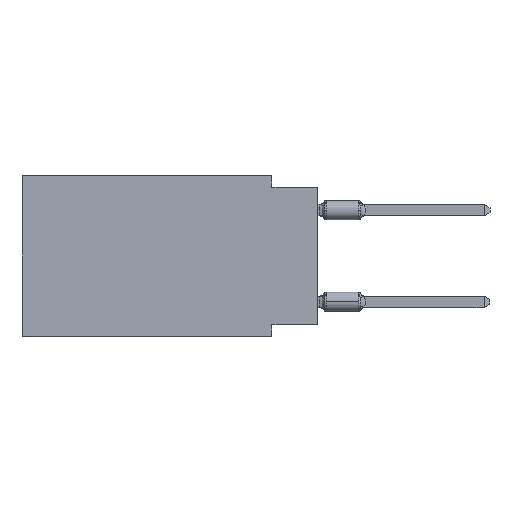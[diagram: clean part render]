
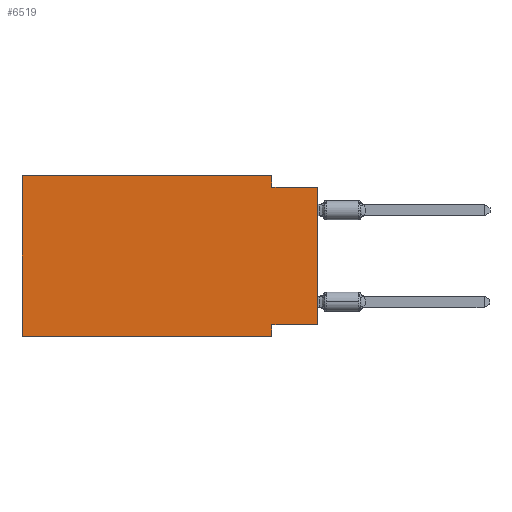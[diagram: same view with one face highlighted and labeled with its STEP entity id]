
A CAD part, left-side view. The second image highlights one B-rep face of the part: STEP entity #6519.
In plain terms, the highlighted planar face has unit normal (-1, 0, 0).
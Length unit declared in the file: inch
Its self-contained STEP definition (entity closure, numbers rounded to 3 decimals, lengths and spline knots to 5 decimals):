
#7 = PLANE ( 'NONE',  #6717 ) ;
#871 = ORIENTED_EDGE ( 'NONE', *, *, #10313, .F. ) ;
#1199 = EDGE_CURVE ( 'NONE', #1504, #3100, #9856, .T. ) ;
#1211 = DIRECTION ( 'NONE',  ( 0., 0., -1. ) ) ;
#1282 = CARTESIAN_POINT ( 'NONE',  ( 0., 0.1, -0.025 ) ) ;
#1340 = VERTEX_POINT ( 'NONE', #2912 ) ;
#1504 = VERTEX_POINT ( 'NONE', #16061 ) ;
#1903 = VECTOR ( 'NONE', #5912, 39.37008 ) ;
#2003 = ORIENTED_EDGE ( 'NONE', *, *, #5111, .F. ) ;
#2334 = EDGE_CURVE ( 'NONE', #6567, #9020, #13738, .T. ) ;
#2909 = EDGE_CURVE ( 'NONE', #7419, #9020, #5508, .T. ) ;
#2912 = CARTESIAN_POINT ( 'NONE',  ( 0., 0.1, -0.35 ) ) ;
#3045 = VECTOR ( 'NONE', #1211, 39.37008 ) ;
#3100 = VERTEX_POINT ( 'NONE', #3592 ) ;
#3111 = CARTESIAN_POINT ( 'NONE',  ( 0., 0., -0.025 ) ) ;
#3592 = CARTESIAN_POINT ( 'NONE',  ( 0., 0.645, 0. ) ) ;
#4078 = CARTESIAN_POINT ( 'NONE',  ( 0., 0.1, 0. ) ) ;
#4549 = CARTESIAN_POINT ( 'NONE',  ( 0., 0.1, 0. ) ) ;
#4563 = DIRECTION ( 'NONE',  ( 0., 0., 1. ) ) ;
#5111 = EDGE_CURVE ( 'NONE', #5443, #1340, #11611, .T. ) ;
#5132 = CARTESIAN_POINT ( 'NONE',  ( 0., 0.1, -0.35 ) ) ;
#5264 = CARTESIAN_POINT ( 'NONE',  ( 0., 0., -0.325 ) ) ;
#5443 = VERTEX_POINT ( 'NONE', #11038 ) ;
#5446 = VECTOR ( 'NONE', #6597, 39.37008 ) ;
#5503 = ORIENTED_EDGE ( 'NONE', *, *, #1199, .F. ) ;
#5508 = LINE ( 'NONE', #14530, #12992 ) ;
#5824 = LINE ( 'NONE', #4549, #1903 ) ;
#5912 = DIRECTION ( 'NONE',  ( 0., 0., -1. ) ) ;
#5937 = VECTOR ( 'NONE', #4563, 39.37008 ) ;
#6387 = DIRECTION ( 'NONE',  ( 0., 1., 0. ) ) ;
#6519 = ADVANCED_FACE ( 'NONE', ( #7775 ), #7, .F. ) ;
#6564 = CARTESIAN_POINT ( 'NONE',  ( 0., 0.645, 0. ) ) ;
#6567 = VERTEX_POINT ( 'NONE', #1282 ) ;
#6597 = DIRECTION ( 'NONE',  ( 0., -1., 0. ) ) ;
#6717 = AXIS2_PLACEMENT_3D ( 'NONE', #6564, #14128, #11755 ) ;
#6775 = ORIENTED_EDGE ( 'NONE', *, *, #2909, .T. ) ;
#6817 = VECTOR ( 'NONE', #13650, 39.37008 ) ;
#7230 = CARTESIAN_POINT ( 'NONE',  ( 0., 0., -0.325 ) ) ;
#7419 = VERTEX_POINT ( 'NONE', #7230 ) ;
#7745 = ORIENTED_EDGE ( 'NONE', *, *, #12721, .F. ) ;
#7775 = FACE_OUTER_BOUND ( 'NONE', #9395, .T. ) ;
#8275 = VECTOR ( 'NONE', #6387, 39.37008 ) ;
#9020 = VERTEX_POINT ( 'NONE', #14349 ) ;
#9084 = LINE ( 'NONE', #10265, #5446 ) ;
#9225 = LINE ( 'NONE', #10323, #15230 ) ;
#9395 = EDGE_LOOP ( 'NONE', ( #6775, #15215, #7745, #12127, #5503, #9955, #2003, #871 ) ) ;
#9846 = EDGE_CURVE ( 'NONE', #3100, #13721, #9225, .T. ) ;
#9856 = LINE ( 'NONE', #11300, #5937 ) ;
#9955 = ORIENTED_EDGE ( 'NONE', *, *, #12815, .T. ) ;
#10228 = LINE ( 'NONE', #5264, #8275 ) ;
#10265 = CARTESIAN_POINT ( 'NONE',  ( 0., 0.645, -0.35 ) ) ;
#10313 = EDGE_CURVE ( 'NONE', #7419, #5443, #10228, .T. ) ;
#10323 = CARTESIAN_POINT ( 'NONE',  ( 0., 0.645, 0. ) ) ;
#10660 = DIRECTION ( 'NONE',  ( 0., -1., 0. ) ) ;
#11038 = CARTESIAN_POINT ( 'NONE',  ( 0., 0.1, -0.325 ) ) ;
#11300 = CARTESIAN_POINT ( 'NONE',  ( 0., 0.645, 0. ) ) ;
#11611 = LINE ( 'NONE', #5132, #3045 ) ;
#11755 = DIRECTION ( 'NONE',  ( 0., 0., -1. ) ) ;
#12127 = ORIENTED_EDGE ( 'NONE', *, *, #9846, .F. ) ;
#12721 = EDGE_CURVE ( 'NONE', #13721, #6567, #5824, .T. ) ;
#12815 = EDGE_CURVE ( 'NONE', #1504, #1340, #9084, .T. ) ;
#12992 = VECTOR ( 'NONE', #13090, 39.37008 ) ;
#13090 = DIRECTION ( 'NONE',  ( 0., 0., 1. ) ) ;
#13650 = DIRECTION ( 'NONE',  ( 0., -1., 0. ) ) ;
#13721 = VERTEX_POINT ( 'NONE', #4078 ) ;
#13738 = LINE ( 'NONE', #3111, #6817 ) ;
#14128 = DIRECTION ( 'NONE',  ( 1., 0., 0. ) ) ;
#14349 = CARTESIAN_POINT ( 'NONE',  ( 0., 0., -0.025 ) ) ;
#14530 = CARTESIAN_POINT ( 'NONE',  ( 0., 0., 0. ) ) ;
#15215 = ORIENTED_EDGE ( 'NONE', *, *, #2334, .F. ) ;
#15230 = VECTOR ( 'NONE', #10660, 39.37008 ) ;
#16061 = CARTESIAN_POINT ( 'NONE',  ( 0., 0.645, -0.35 ) ) ;
